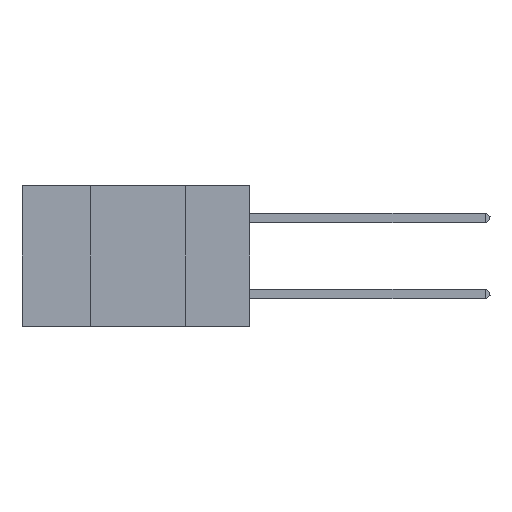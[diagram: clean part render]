
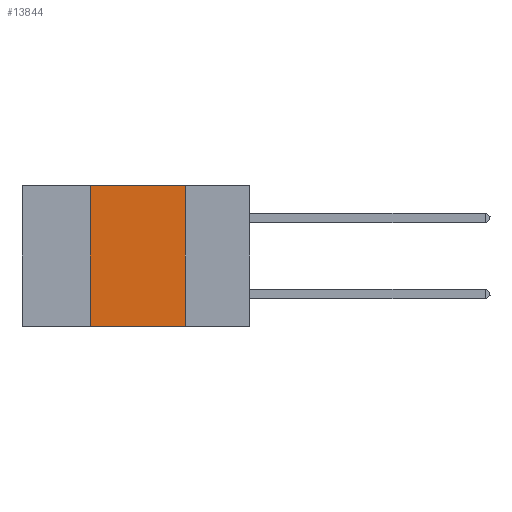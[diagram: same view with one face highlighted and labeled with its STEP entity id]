
A CAD part, left-side view. The second image highlights one B-rep face of the part: STEP entity #13844.
In plain terms, the highlighted planar face has unit normal (-1, 0, 0).
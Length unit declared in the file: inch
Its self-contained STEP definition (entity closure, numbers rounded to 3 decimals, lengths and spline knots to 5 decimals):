
#810 = PLANE ( 'NONE',  #35855 ) ;
#1359 = VECTOR ( 'NONE', #23549, 39.37008 ) ;
#2378 = LINE ( 'NONE', #9149, #35200 ) ;
#4550 = CARTESIAN_POINT ( 'NONE',  ( 0., 0.42, 0. ) ) ;
#5269 = CARTESIAN_POINT ( 'NONE',  ( 0., 0.42, -0.37 ) ) ;
#6200 = CARTESIAN_POINT ( 'NONE',  ( 0., 0.42, 0. ) ) ;
#8155 = VERTEX_POINT ( 'NONE', #5269 ) ;
#8519 = VERTEX_POINT ( 'NONE', #20426 ) ;
#8848 = EDGE_CURVE ( 'NONE', #8519, #26749, #2378, .T. ) ;
#8877 = LINE ( 'NONE', #19914, #28112 ) ;
#9149 = CARTESIAN_POINT ( 'NONE',  ( 0., 0.17, 0. ) ) ;
#9583 = EDGE_CURVE ( 'NONE', #8155, #26749, #26300, .T. ) ;
#10494 = ORIENTED_EDGE ( 'NONE', *, *, #9583, .T. ) ;
#11428 = CARTESIAN_POINT ( 'NONE',  ( 0., 0.6, -0.37 ) ) ;
#13844 = ADVANCED_FACE ( 'NONE', ( #24966 ), #810, .F. ) ;
#14458 = EDGE_LOOP ( 'NONE', ( #28842, #28037, #30389, #10494 ) ) ;
#16315 = DIRECTION ( 'NONE',  ( 0., 0., 1. ) ) ;
#16737 = DIRECTION ( 'NONE',  ( 0., -1., 0. ) ) ;
#17296 = EDGE_CURVE ( 'NONE', #26421, #8519, #8877, .T. ) ;
#18973 = CARTESIAN_POINT ( 'NONE',  ( 0., 0.6, 0. ) ) ;
#19062 = CARTESIAN_POINT ( 'NONE',  ( 0., 0.17, -0.37 ) ) ;
#19914 = CARTESIAN_POINT ( 'NONE',  ( 0., 0.6, 0. ) ) ;
#20181 = EDGE_CURVE ( 'NONE', #8155, #26421, #27449, .T. ) ;
#20426 = CARTESIAN_POINT ( 'NONE',  ( 0., 0.17, 0. ) ) ;
#23549 = DIRECTION ( 'NONE',  ( 0., -1., 0. ) ) ;
#24966 = FACE_OUTER_BOUND ( 'NONE', #14458, .T. ) ;
#26300 = LINE ( 'NONE', #11428, #1359 ) ;
#26421 = VERTEX_POINT ( 'NONE', #6200 ) ;
#26749 = VERTEX_POINT ( 'NONE', #19062 ) ;
#27449 = LINE ( 'NONE', #4550, #35911 ) ;
#27629 = DIRECTION ( 'NONE',  ( 0., 0., -1. ) ) ;
#28037 = ORIENTED_EDGE ( 'NONE', *, *, #17296, .F. ) ;
#28112 = VECTOR ( 'NONE', #16737, 39.37008 ) ;
#28842 = ORIENTED_EDGE ( 'NONE', *, *, #8848, .F. ) ;
#30389 = ORIENTED_EDGE ( 'NONE', *, *, #20181, .F. ) ;
#32575 = DIRECTION ( 'NONE',  ( 0., 0., -1. ) ) ;
#34681 = DIRECTION ( 'NONE',  ( 1., 0., 0. ) ) ;
#35200 = VECTOR ( 'NONE', #27629, 39.37008 ) ;
#35855 = AXIS2_PLACEMENT_3D ( 'NONE', #18973, #34681, #32575 ) ;
#35911 = VECTOR ( 'NONE', #16315, 39.37008 ) ;
